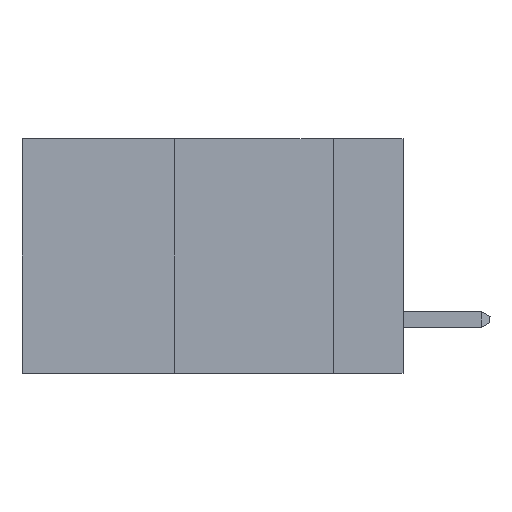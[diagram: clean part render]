
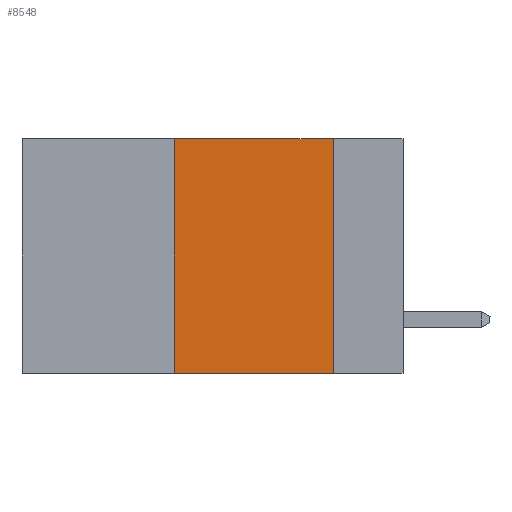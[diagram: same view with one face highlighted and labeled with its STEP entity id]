
A CAD part, left-side view. The second image highlights one B-rep face of the part: STEP entity #8548.
In plain terms, the highlighted planar face has unit normal (-1, 0, 0).
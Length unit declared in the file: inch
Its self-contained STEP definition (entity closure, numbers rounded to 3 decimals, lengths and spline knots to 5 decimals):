
#106 = DIRECTION ( 'NONE',  ( 0., 0., 1. ) ) ;
#293 = CARTESIAN_POINT ( 'NONE',  ( 0., 0.11, 0. ) ) ;
#1061 = VECTOR ( 'NONE', #106, 39.37008 ) ;
#1062 = ORIENTED_EDGE ( 'NONE', *, *, #7656, .F. ) ;
#1573 = LINE ( 'NONE', #1668, #1992 ) ;
#1668 = CARTESIAN_POINT ( 'NONE',  ( 0., 0.6, 0. ) ) ;
#1841 = VERTEX_POINT ( 'NONE', #15226 ) ;
#1843 = VECTOR ( 'NONE', #4946, 39.37008 ) ;
#1992 = VECTOR ( 'NONE', #17704, 39.37008 ) ;
#3461 = CARTESIAN_POINT ( 'NONE',  ( 0., 0.36, 0. ) ) ;
#3787 = EDGE_CURVE ( 'NONE', #1841, #7435, #16784, .T. ) ;
#4532 = VERTEX_POINT ( 'NONE', #12623 ) ;
#4537 = LINE ( 'NONE', #5893, #12718 ) ;
#4946 = DIRECTION ( 'NONE',  ( 0., 0., -1. ) ) ;
#5283 = FACE_OUTER_BOUND ( 'NONE', #10501, .T. ) ;
#5893 = CARTESIAN_POINT ( 'NONE',  ( 0., 0.6, -0.37 ) ) ;
#6731 = AXIS2_PLACEMENT_3D ( 'NONE', #14135, #13861, #8116 ) ;
#6795 = EDGE_CURVE ( 'NONE', #1841, #4532, #4537, .T. ) ;
#7435 = VERTEX_POINT ( 'NONE', #17128 ) ;
#7656 = EDGE_CURVE ( 'NONE', #17432, #4532, #17888, .T. ) ;
#8116 = DIRECTION ( 'NONE',  ( 0., 0., -1. ) ) ;
#8548 = ADVANCED_FACE ( 'NONE', ( #5283 ), #10903, .F. ) ;
#10501 = EDGE_LOOP ( 'NONE', ( #1062, #16341, #11453, #11481 ) ) ;
#10903 = PLANE ( 'NONE',  #6731 ) ;
#11453 = ORIENTED_EDGE ( 'NONE', *, *, #3787, .F. ) ;
#11481 = ORIENTED_EDGE ( 'NONE', *, *, #6795, .T. ) ;
#11797 = DIRECTION ( 'NONE',  ( 0., -1., 0. ) ) ;
#12447 = EDGE_CURVE ( 'NONE', #7435, #17432, #1573, .T. ) ;
#12623 = CARTESIAN_POINT ( 'NONE',  ( 0., 0.11, -0.37 ) ) ;
#12718 = VECTOR ( 'NONE', #11797, 39.37008 ) ;
#13861 = DIRECTION ( 'NONE',  ( 1., 0., 0. ) ) ;
#14135 = CARTESIAN_POINT ( 'NONE',  ( 0., 0.6, 0. ) ) ;
#15226 = CARTESIAN_POINT ( 'NONE',  ( 0., 0.36, -0.37 ) ) ;
#16341 = ORIENTED_EDGE ( 'NONE', *, *, #12447, .F. ) ;
#16784 = LINE ( 'NONE', #3461, #1061 ) ;
#17128 = CARTESIAN_POINT ( 'NONE',  ( 0., 0.36, 0. ) ) ;
#17432 = VERTEX_POINT ( 'NONE', #293 ) ;
#17704 = DIRECTION ( 'NONE',  ( 0., -1., 0. ) ) ;
#17888 = LINE ( 'NONE', #18262, #1843 ) ;
#18262 = CARTESIAN_POINT ( 'NONE',  ( 0., 0.11, 0. ) ) ;
